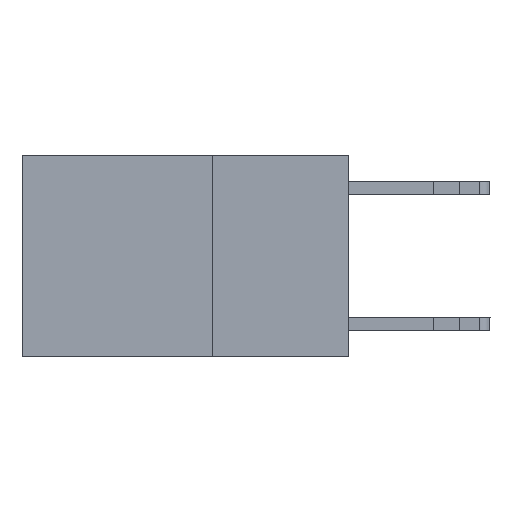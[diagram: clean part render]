
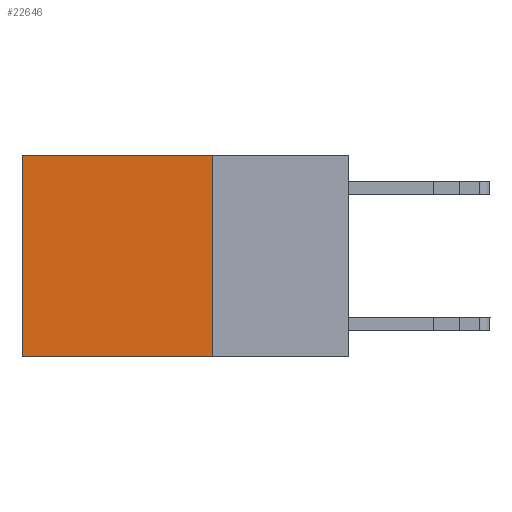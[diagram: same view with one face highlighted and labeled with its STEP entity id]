
A CAD part, left-side view. The second image highlights one B-rep face of the part: STEP entity #22646.
In plain terms, the highlighted planar face has unit normal (-1, 0, 0).
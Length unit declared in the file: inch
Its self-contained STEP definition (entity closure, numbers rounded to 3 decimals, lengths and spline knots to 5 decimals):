
#192 = EDGE_CURVE ( 'NONE', #5540, #13572, #2003, .T. ) ;
#674 = CARTESIAN_POINT ( 'NONE',  ( 0.2625, 0.25, -0.37 ) ) ;
#1573 = CARTESIAN_POINT ( 'NONE',  ( 0.2625, 0.6, 0. ) ) ;
#1829 = EDGE_LOOP ( 'NONE', ( #13035, #25865, #24002, #10397 ) ) ;
#2003 = LINE ( 'NONE', #8940, #12814 ) ;
#3031 = DIRECTION ( 'NONE',  ( 0., 1., 0. ) ) ;
#3531 = EDGE_CURVE ( 'NONE', #5540, #5297, #16354, .T. ) ;
#3765 = DIRECTION ( 'NONE',  ( 0., 0., -1. ) ) ;
#5297 = VERTEX_POINT ( 'NONE', #7123 ) ;
#5540 = VERTEX_POINT ( 'NONE', #22848 ) ;
#6066 = VECTOR ( 'NONE', #3765, 39.37008 ) ;
#6155 = VERTEX_POINT ( 'NONE', #9295 ) ;
#7123 = CARTESIAN_POINT ( 'NONE',  ( 0.2625, 0.6, 0. ) ) ;
#7393 = AXIS2_PLACEMENT_3D ( 'NONE', #22561, #9677, #24719 ) ;
#7479 = PLANE ( 'NONE',  #7393 ) ;
#8856 = EDGE_CURVE ( 'NONE', #13572, #6155, #27264, .T. ) ;
#8940 = CARTESIAN_POINT ( 'NONE',  ( 0.2625, 0.25, 0. ) ) ;
#9295 = CARTESIAN_POINT ( 'NONE',  ( 0.2625, 0.6, -0.37 ) ) ;
#9677 = DIRECTION ( 'NONE',  ( 1., 0., 0. ) ) ;
#9865 = CARTESIAN_POINT ( 'NONE',  ( 0.2625, 0.25, 0. ) ) ;
#10397 = ORIENTED_EDGE ( 'NONE', *, *, #3531, .T. ) ;
#11081 = FACE_OUTER_BOUND ( 'NONE', #1829, .T. ) ;
#12814 = VECTOR ( 'NONE', #13256, 39.37008 ) ;
#13035 = ORIENTED_EDGE ( 'NONE', *, *, #21668, .T. ) ;
#13256 = DIRECTION ( 'NONE',  ( 0., 0., -1. ) ) ;
#13572 = VERTEX_POINT ( 'NONE', #674 ) ;
#15937 = CARTESIAN_POINT ( 'NONE',  ( 0.2625, 0.25, -0.37 ) ) ;
#16354 = LINE ( 'NONE', #9865, #22057 ) ;
#18210 = LINE ( 'NONE', #1573, #6066 ) ;
#21668 = EDGE_CURVE ( 'NONE', #5297, #6155, #18210, .T. ) ;
#22057 = VECTOR ( 'NONE', #24910, 39.37008 ) ;
#22561 = CARTESIAN_POINT ( 'NONE',  ( 0.2625, 0.25, 0. ) ) ;
#22646 = ADVANCED_FACE ( 'NONE', ( #11081 ), #7479, .F. ) ;
#22848 = CARTESIAN_POINT ( 'NONE',  ( 0.2625, 0.25, 0. ) ) ;
#24002 = ORIENTED_EDGE ( 'NONE', *, *, #192, .F. ) ;
#24719 = DIRECTION ( 'NONE',  ( 0., 0., -1. ) ) ;
#24910 = DIRECTION ( 'NONE',  ( 0., 1., 0. ) ) ;
#25865 = ORIENTED_EDGE ( 'NONE', *, *, #8856, .F. ) ;
#26594 = VECTOR ( 'NONE', #3031, 39.37008 ) ;
#27264 = LINE ( 'NONE', #15937, #26594 ) ;
